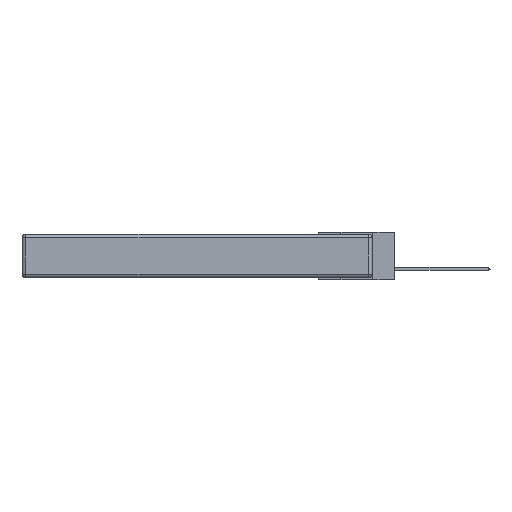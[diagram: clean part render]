
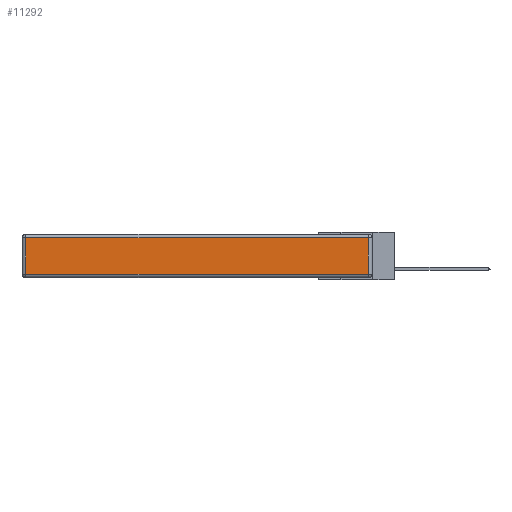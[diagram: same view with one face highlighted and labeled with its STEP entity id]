
A CAD part, left-side view. The second image highlights one B-rep face of the part: STEP entity #11292.
In plain terms, the highlighted planar face has unit normal (-1, 0, 0).
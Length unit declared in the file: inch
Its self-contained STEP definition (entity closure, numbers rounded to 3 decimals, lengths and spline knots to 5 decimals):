
#116 = CARTESIAN_POINT ( 'NONE',  ( 0., 2.72, -0.343 ) ) ;
#1590 = EDGE_LOOP ( 'NONE', ( #15083, #16117, #13892, #14561 ) ) ;
#2614 = LINE ( 'NONE', #116, #8124 ) ;
#3062 = CARTESIAN_POINT ( 'NONE',  ( 0., 0.03, -0.343 ) ) ;
#3134 = DIRECTION ( 'NONE',  ( -1., 0., 0. ) ) ;
#4488 = DIRECTION ( 'NONE',  ( 0., -1., 0. ) ) ;
#4740 = CARTESIAN_POINT ( 'NONE',  ( 0., 0.03, -0.313 ) ) ;
#5032 = VECTOR ( 'NONE', #5775, 39.37008 ) ;
#5172 = EDGE_CURVE ( 'NONE', #9909, #14821, #2614, .T. ) ;
#5454 = VECTOR ( 'NONE', #4488, 39.37008 ) ;
#5666 = PLANE ( 'NONE',  #17700 ) ;
#5704 = VERTEX_POINT ( 'NONE', #4740 ) ;
#5775 = DIRECTION ( 'NONE',  ( 0., 0., 1. ) ) ;
#5848 = EDGE_CURVE ( 'NONE', #14821, #5704, #10937, .T. ) ;
#6901 = CARTESIAN_POINT ( 'NONE',  ( 0., 2.72, -0.313 ) ) ;
#8049 = CARTESIAN_POINT ( 'NONE',  ( 0., 2.75, -0.03 ) ) ;
#8124 = VECTOR ( 'NONE', #9957, 39.37008 ) ;
#9657 = EDGE_CURVE ( 'NONE', #5704, #10322, #14493, .T. ) ;
#9785 = VECTOR ( 'NONE', #12410, 39.37008 ) ;
#9909 = VERTEX_POINT ( 'NONE', #10440 ) ;
#9957 = DIRECTION ( 'NONE',  ( 0., 0., -1. ) ) ;
#10322 = VERTEX_POINT ( 'NONE', #16986 ) ;
#10440 = CARTESIAN_POINT ( 'NONE',  ( 0., 2.72, -0.03 ) ) ;
#10937 = LINE ( 'NONE', #15560, #5454 ) ;
#11292 = ADVANCED_FACE ( 'NONE', ( #13329 ), #5666, .T. ) ;
#11306 = LINE ( 'NONE', #8049, #9785 ) ;
#12410 = DIRECTION ( 'NONE',  ( 0., 1., 0. ) ) ;
#13329 = FACE_OUTER_BOUND ( 'NONE', #1590, .T. ) ;
#13892 = ORIENTED_EDGE ( 'NONE', *, *, #18030, .T. ) ;
#14273 = DIRECTION ( 'NONE',  ( 0., 0., 1. ) ) ;
#14493 = LINE ( 'NONE', #3062, #5032 ) ;
#14561 = ORIENTED_EDGE ( 'NONE', *, *, #5172, .T. ) ;
#14821 = VERTEX_POINT ( 'NONE', #6901 ) ;
#15083 = ORIENTED_EDGE ( 'NONE', *, *, #5848, .T. ) ;
#15560 = CARTESIAN_POINT ( 'NONE',  ( 0., 0., -0.313 ) ) ;
#16117 = ORIENTED_EDGE ( 'NONE', *, *, #9657, .T. ) ;
#16889 = CARTESIAN_POINT ( 'NONE',  ( 0., 0., -0.343 ) ) ;
#16986 = CARTESIAN_POINT ( 'NONE',  ( 0., 0.03, -0.03 ) ) ;
#17700 = AXIS2_PLACEMENT_3D ( 'NONE', #16889, #3134, #14273 ) ;
#18030 = EDGE_CURVE ( 'NONE', #10322, #9909, #11306, .T. ) ;
